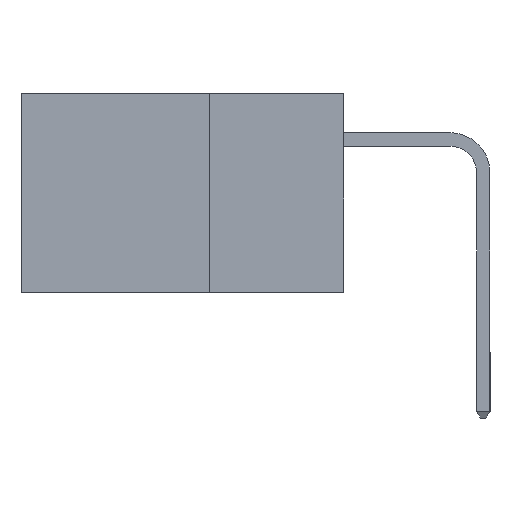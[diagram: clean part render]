
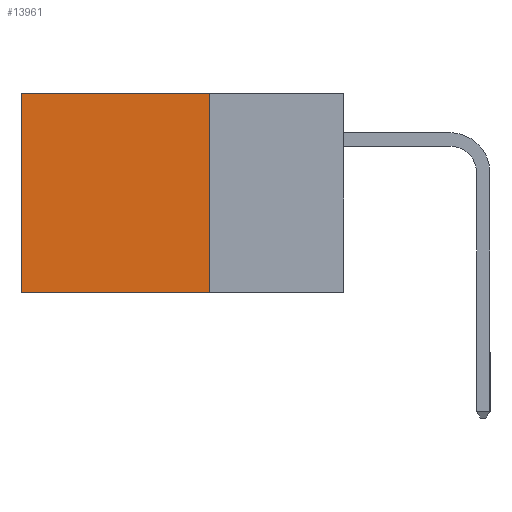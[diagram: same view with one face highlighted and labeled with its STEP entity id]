
A CAD part, left-side view. The second image highlights one B-rep face of the part: STEP entity #13961.
In plain terms, the highlighted planar face has unit normal (-1, 0, 0).
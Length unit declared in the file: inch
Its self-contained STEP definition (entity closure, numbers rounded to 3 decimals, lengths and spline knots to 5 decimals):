
#234 = CARTESIAN_POINT ( 'NONE',  ( 0.298, 0.25, 0. ) ) ;
#1708 = FACE_OUTER_BOUND ( 'NONE', #3212, .T. ) ;
#1840 = CARTESIAN_POINT ( 'NONE',  ( 0.298, 0.6, 0. ) ) ;
#2059 = LINE ( 'NONE', #5660, #18030 ) ;
#2064 = AXIS2_PLACEMENT_3D ( 'NONE', #9834, #12677, #2773 ) ;
#2773 = DIRECTION ( 'NONE',  ( 0., 0., -1. ) ) ;
#2865 = CARTESIAN_POINT ( 'NONE',  ( 0.298, 0.25, 0. ) ) ;
#3212 = EDGE_LOOP ( 'NONE', ( #4470, #13875, #17883, #16919 ) ) ;
#4225 = VERTEX_POINT ( 'NONE', #9019 ) ;
#4470 = ORIENTED_EDGE ( 'NONE', *, *, #14884, .T. ) ;
#4934 = VECTOR ( 'NONE', #15566, 39.37008 ) ;
#5648 = VERTEX_POINT ( 'NONE', #15899 ) ;
#5660 = CARTESIAN_POINT ( 'NONE',  ( 0.298, 0.25, -0.37 ) ) ;
#6186 = EDGE_CURVE ( 'NONE', #11720, #5648, #2059, .T. ) ;
#6916 = CARTESIAN_POINT ( 'NONE',  ( 0.298, 0.25, -0.37 ) ) ;
#7350 = LINE ( 'NONE', #234, #10231 ) ;
#7616 = VECTOR ( 'NONE', #16180, 39.37008 ) ;
#7822 = LINE ( 'NONE', #1840, #7616 ) ;
#8272 = LINE ( 'NONE', #2865, #4934 ) ;
#8580 = DIRECTION ( 'NONE',  ( 0., 1., 0. ) ) ;
#9019 = CARTESIAN_POINT ( 'NONE',  ( 0.298, 0.6, 0. ) ) ;
#9261 = EDGE_CURVE ( 'NONE', #16654, #11720, #8272, .T. ) ;
#9834 = CARTESIAN_POINT ( 'NONE',  ( 0.298, 0.25, 0. ) ) ;
#10231 = VECTOR ( 'NONE', #8580, 39.37008 ) ;
#11195 = DIRECTION ( 'NONE',  ( 0., 1., 0. ) ) ;
#11720 = VERTEX_POINT ( 'NONE', #6916 ) ;
#12677 = DIRECTION ( 'NONE',  ( 1., 0., 0. ) ) ;
#12900 = CARTESIAN_POINT ( 'NONE',  ( 0.298, 0.25, 0. ) ) ;
#13875 = ORIENTED_EDGE ( 'NONE', *, *, #6186, .F. ) ;
#13961 = ADVANCED_FACE ( 'NONE', ( #1708 ), #17215, .F. ) ;
#14884 = EDGE_CURVE ( 'NONE', #4225, #5648, #7822, .T. ) ;
#15566 = DIRECTION ( 'NONE',  ( 0., 0., -1. ) ) ;
#15899 = CARTESIAN_POINT ( 'NONE',  ( 0.298, 0.6, -0.37 ) ) ;
#16180 = DIRECTION ( 'NONE',  ( 0., 0., -1. ) ) ;
#16628 = EDGE_CURVE ( 'NONE', #16654, #4225, #7350, .T. ) ;
#16654 = VERTEX_POINT ( 'NONE', #12900 ) ;
#16919 = ORIENTED_EDGE ( 'NONE', *, *, #16628, .T. ) ;
#17215 = PLANE ( 'NONE',  #2064 ) ;
#17883 = ORIENTED_EDGE ( 'NONE', *, *, #9261, .F. ) ;
#18030 = VECTOR ( 'NONE', #11195, 39.37008 ) ;
